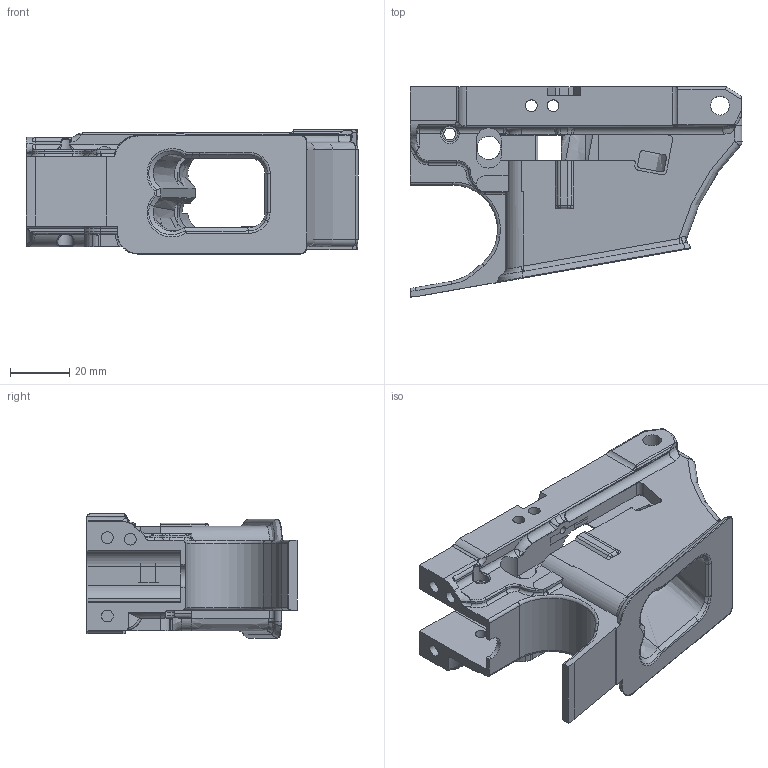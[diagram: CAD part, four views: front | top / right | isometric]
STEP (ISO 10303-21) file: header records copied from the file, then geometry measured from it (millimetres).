
FILE_DESCRIPTION(/* description */ (''),/* implementation_level */ '2;1');
FILE_NAME(/* name */ 'WWSD 9mm Glock Magwell.step',/* time_stamp */ '2020-04-07T01:54:44-05:00',/* author */ (''),/* organization */ (''),/* preprocessor_version */ 'ST-DEVELOPER v18',/* originating_system */ 'Autodesk Translation Framework v8.12.0.6',/* authorisation */ '');
FILE_SCHEMA (('AUTOMOTIVE_DESIGN { 1 0 10303 214 3 1 1 }'));
Length unit declared in the file: millimetre
Products named in the file (1): (Unsaved)
Bounding box: 112.45 x 71.13 x 42.01 mm (x, y, z)
Volume: 117443.5 mm3; surface area: 37104.5 mm2
Topology: 1 solids, 5 shells, 488 faces, 1356 edges, 873 vertices
Faces by surface type: plane 160, bspline 151, cylinder 145, torus 31, cone 1
Full cylindrical faces by diameter (mm): 2.54 x2, 3.962 x2, 4 x9, 5.389 x1, 5.394 x1, 6.375 x2, 7.938 x1
Entity records: 22827 total; most frequent: CARTESIAN_POINT 11202, ORIENTED_EDGE 2704, DIRECTION 1995, EDGE_CURVE 1352, VERTEX_POINT 873, AXIS2_PLACEMENT_3D 707, LINE 581, VECTOR 581
